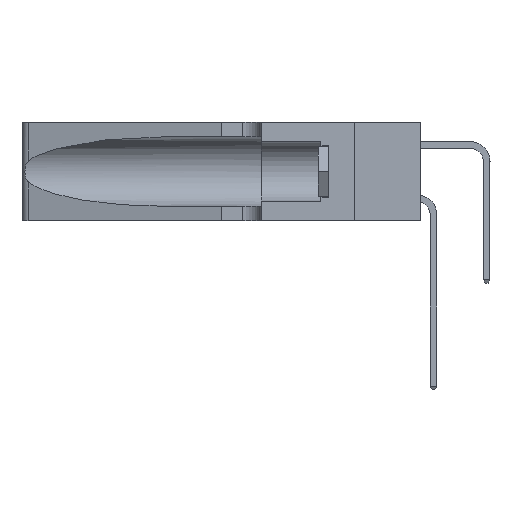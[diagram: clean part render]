
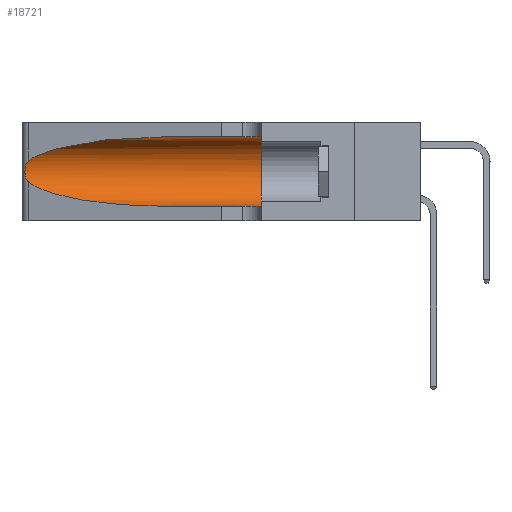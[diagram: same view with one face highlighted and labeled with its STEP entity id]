
A CAD part, left-side view. The second image highlights one B-rep face of the part: STEP entity #18721.
In plain terms, the highlighted cylindrical face has radius 3.308 mm (diameter 6.617 mm), a partial arc.
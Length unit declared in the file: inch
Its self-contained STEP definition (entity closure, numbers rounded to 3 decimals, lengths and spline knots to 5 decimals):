
#709 = CYLINDRICAL_SURFACE ( 'NONE', #5060, 0.13025 ) ;
#2179 = DIRECTION ( 'NONE',  ( 0., -1., 0. ) ) ;
#2239 = CARTESIAN_POINT ( 'NONE',  ( 0.1305, 0.72297, 0.31525 ) ) ;
#2254 = DIRECTION ( 'NONE',  ( 0., 0., -1. ) ) ;
#2292 = EDGE_LOOP ( 'NONE', ( #24138, #18620, #37455, #31086, #15128, #9537 ) ) ;
#2497 = CARTESIAN_POINT ( 'NONE',  ( 0.25856, 1.23593, 0.16098 ) ) ;
#3110 =( BOUNDED_CURVE ( )  B_SPLINE_CURVE ( 3, ( #31558, #9134, #15664, #37837 ),
 .UNSPECIFIED., .F., .T. ) 
 B_SPLINE_CURVE_WITH_KNOTS ( ( 4, 4 ),
 ( 3.44316, 4.71239 ),
 .UNSPECIFIED. ) 
 CURVE ( )  GEOMETRIC_REPRESENTATION_ITEM ( )  RATIONAL_B_SPLINE_CURVE ( ( 1., 0.87, 0.87, 1. ) ) 
 REPRESENTATION_ITEM ( '' )  );
#4415 = VERTEX_POINT ( 'NONE', #2239 ) ;
#4646 = AXIS2_PLACEMENT_3D ( 'NONE', #17810, #39930, #21040 ) ;
#4810 = EDGE_CURVE ( 'NONE', #4415, #30336, #6257, .T. ) ;
#5060 = AXIS2_PLACEMENT_3D ( 'NONE', #21676, #34274, #2254 ) ;
#5667 = VERTEX_POINT ( 'NONE', #18057 ) ;
#5784 = CARTESIAN_POINT ( 'NONE',  ( 0.25639, 1.23186, 0.15144 ) ) ;
#6155 = EDGE_CURVE ( 'NONE', #19682, #36461, #17734, .T. ) ;
#6257 =( BOUNDED_CURVE ( )  B_SPLINE_CURVE ( 3, ( #14018, #29950, #17280, #39411 ),
 .UNSPECIFIED., .F., .F. ) 
 B_SPLINE_CURVE_WITH_KNOTS ( ( 4, 4 ),
 ( 1.5708, 2.84003 ),
 .UNSPECIFIED. ) 
 CURVE ( )  GEOMETRIC_REPRESENTATION_ITEM ( )  RATIONAL_B_SPLINE_CURVE ( ( 1., 0.87, 0.87, 1. ) ) 
 REPRESENTATION_ITEM ( '' )  );
#9059 = CARTESIAN_POINT ( 'NONE',  ( 0.25487, 1.22718, 0.14631 ) ) ;
#9134 = CARTESIAN_POINT ( 'NONE',  ( 0.2373, 1.15595, 0.08982 ) ) ;
#9537 = ORIENTED_EDGE ( 'NONE', *, *, #30372, .F. ) ;
#12143 = CARTESIAN_POINT ( 'NONE',  ( 0.25639, 1.23184, 0.21858 ) ) ;
#14018 = CARTESIAN_POINT ( 'NONE',  ( 0.1305, 0.72297, 0.31525 ) ) ;
#14337 = EDGE_CURVE ( 'NONE', #5667, #19682, #3110, .T. ) ;
#15128 = ORIENTED_EDGE ( 'NONE', *, *, #33590, .F. ) ;
#15442 = CARTESIAN_POINT ( 'NONE',  ( 0.25854, 1.2359, 0.20912 ) ) ;
#15664 = CARTESIAN_POINT ( 'NONE',  ( 0.18966, 0.96281, 0.05475 ) ) ;
#17280 = CARTESIAN_POINT ( 'NONE',  ( 0.2373, 1.15595, 0.28018 ) ) ;
#17734 = LINE ( 'NONE', #28006, #40971 ) ;
#17810 = CARTESIAN_POINT ( 'NONE',  ( 0.1305, 0.35, 0.185 ) ) ;
#17965 = FACE_OUTER_BOUND ( 'NONE', #2292, .T. ) ;
#18057 = CARTESIAN_POINT ( 'NONE',  ( 0.25487, 1.22718, 0.14631 ) ) ;
#18620 = ORIENTED_EDGE ( 'NONE', *, *, #39008, .T. ) ;
#18675 = CARTESIAN_POINT ( 'NONE',  ( 0.26075, 1.23896, 0.19203 ) ) ;
#18721 = ADVANCED_FACE ( 'NONE', ( #17965 ), #709, .F. ) ;
#19453 = CARTESIAN_POINT ( 'NONE',  ( 0.1305, 0.35, 0.05475 ) ) ;
#19488 = B_SPLINE_CURVE_WITH_KNOTS ( 'NONE', 3,
 ( #28169, #31343, #12143, #34492, #15442, #37637, #18675, #40760, #21908, #2497, #25128, #5784, #28300, #9059 ),
 .UNSPECIFIED., .F., .F.,
 ( 4, 2, 2, 2, 2, 2, 4 ),
 ( 0., 0.00027, 0.00053, 0.00107, 0.0016, 0.00187, 0.00214 ),
 .UNSPECIFIED. ) ;
#19516 = LINE ( 'NONE', #26003, #35385 ) ;
#19682 = VERTEX_POINT ( 'NONE', #29130 ) ;
#20858 = VERTEX_POINT ( 'NONE', #22082 ) ;
#21040 = DIRECTION ( 'NONE',  ( 0., 0., 1. ) ) ;
#21676 = CARTESIAN_POINT ( 'NONE',  ( 0.1305, 1.61858, 0.185 ) ) ;
#21708 = CIRCLE ( 'NONE', #4646, 0.13025 ) ;
#21908 = CARTESIAN_POINT ( 'NONE',  ( 0.26017, 1.23833, 0.17102 ) ) ;
#22082 = CARTESIAN_POINT ( 'NONE',  ( 0.1305, 0.35, 0.31525 ) ) ;
#24138 = ORIENTED_EDGE ( 'NONE', *, *, #4810, .T. ) ;
#25128 = CARTESIAN_POINT ( 'NONE',  ( 0.25789, 1.23486, 0.15765 ) ) ;
#26003 = CARTESIAN_POINT ( 'NONE',  ( 0.1305, 1.61858, 0.31525 ) ) ;
#28006 = CARTESIAN_POINT ( 'NONE',  ( 0.1305, 1.61858, 0.05475 ) ) ;
#28169 = CARTESIAN_POINT ( 'NONE',  ( 0.25487, 1.22718, 0.22369 ) ) ;
#28300 = CARTESIAN_POINT ( 'NONE',  ( 0.25555, 1.22993, 0.14849 ) ) ;
#29130 = CARTESIAN_POINT ( 'NONE',  ( 0.1305, 0.72297, 0.05475 ) ) ;
#29187 = DIRECTION ( 'NONE',  ( 0., -1., 0. ) ) ;
#29950 = CARTESIAN_POINT ( 'NONE',  ( 0.18966, 0.96281, 0.31525 ) ) ;
#30336 = VERTEX_POINT ( 'NONE', #35237 ) ;
#30372 = EDGE_CURVE ( 'NONE', #4415, #20858, #19516, .T. ) ;
#31086 = ORIENTED_EDGE ( 'NONE', *, *, #6155, .T. ) ;
#31343 = CARTESIAN_POINT ( 'NONE',  ( 0.25555, 1.22994, 0.2215 ) ) ;
#31558 = CARTESIAN_POINT ( 'NONE',  ( 0.25487, 1.22718, 0.14631 ) ) ;
#33590 = EDGE_CURVE ( 'NONE', #20858, #36461, #21708, .T. ) ;
#34274 = DIRECTION ( 'NONE',  ( 0., -1., 0. ) ) ;
#34492 = CARTESIAN_POINT ( 'NONE',  ( 0.25787, 1.23484, 0.2124 ) ) ;
#35237 = CARTESIAN_POINT ( 'NONE',  ( 0.25487, 1.22718, 0.22369 ) ) ;
#35385 = VECTOR ( 'NONE', #29187, 39.37008 ) ;
#36461 = VERTEX_POINT ( 'NONE', #19453 ) ;
#37455 = ORIENTED_EDGE ( 'NONE', *, *, #14337, .T. ) ;
#37637 = CARTESIAN_POINT ( 'NONE',  ( 0.26018, 1.23835, 0.19895 ) ) ;
#37837 = CARTESIAN_POINT ( 'NONE',  ( 0.1305, 0.72297, 0.05475 ) ) ;
#39008 = EDGE_CURVE ( 'NONE', #30336, #5667, #19488, .T. ) ;
#39411 = CARTESIAN_POINT ( 'NONE',  ( 0.25487, 1.22718, 0.22369 ) ) ;
#39930 = DIRECTION ( 'NONE',  ( 0., 1., 0. ) ) ;
#40760 = CARTESIAN_POINT ( 'NONE',  ( 0.26075, 1.23896, 0.178 ) ) ;
#40971 = VECTOR ( 'NONE', #2179, 39.37008 ) ;
